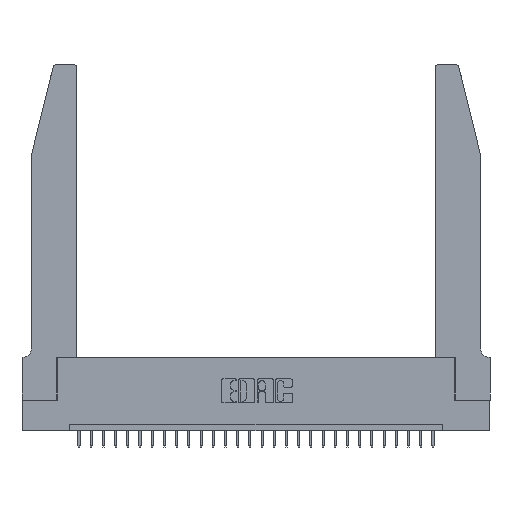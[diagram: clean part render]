
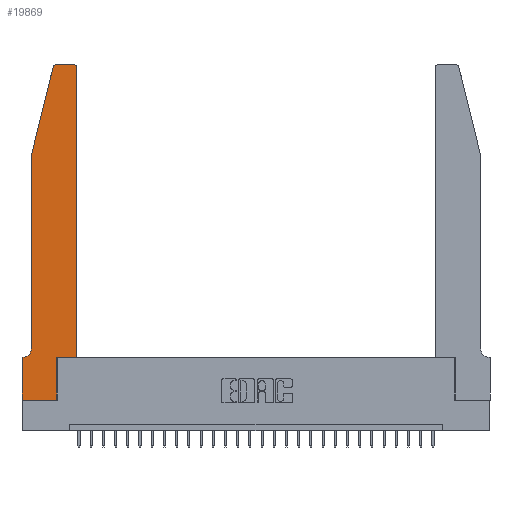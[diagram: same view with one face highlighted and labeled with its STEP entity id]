
A CAD part, top view. The second image highlights one B-rep face of the part: STEP entity #19869.
In plain terms, the highlighted planar face has unit normal (0, 0, 1).
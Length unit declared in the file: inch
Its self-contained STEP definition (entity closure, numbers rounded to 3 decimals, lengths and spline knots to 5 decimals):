
#44 = DIRECTION ( 'NONE',  ( 0., 0., 1. ) ) ;
#77 = AXIS2_PLACEMENT_3D ( 'NONE', #23384, #14602, #3394 ) ;
#98 = VECTOR ( 'NONE', #6298, 39.37008 ) ;
#285 = EDGE_CURVE ( 'NONE', #10634, #1515, #1012, .T. ) ;
#1012 = LINE ( 'NONE', #17188, #25601 ) ;
#1512 = EDGE_CURVE ( 'NONE', #27253, #10078, #5974, .T. ) ;
#1515 = VERTEX_POINT ( 'NONE', #17982 ) ;
#2240 = CARTESIAN_POINT ( 'NONE',  ( 0.284, 2.72, 0.37 ) ) ;
#2306 = ORIENTED_EDGE ( 'NONE', *, *, #8383, .T. ) ;
#2870 = CARTESIAN_POINT ( 'NONE',  ( 0.0055, 0.42, 0.37 ) ) ;
#3179 = DIRECTION ( 'NONE',  ( -0.239, -0.971, 0. ) ) ;
#3394 = DIRECTION ( 'NONE',  ( 1., 0., 0. ) ) ;
#3932 = LINE ( 'NONE', #19424, #98 ) ;
#4130 = ORIENTED_EDGE ( 'NONE', *, *, #18669, .T. ) ;
#4295 = CARTESIAN_POINT ( 'NONE',  ( 0.2865, 0.35, 0.37 ) ) ;
#4354 = ORIENTED_EDGE ( 'NONE', *, *, #24389, .T. ) ;
#4366 = EDGE_LOOP ( 'NONE', ( #11597, #15794, #4354, #13078, #4130, #20273, #5913, #2306, #17979, #25683, #22685, #17369 ) ) ;
#4673 = LINE ( 'NONE', #11327, #28421 ) ;
#5913 = ORIENTED_EDGE ( 'NONE', *, *, #285, .T. ) ;
#5974 = CIRCLE ( 'NONE', #15387, 0.03 ) ;
#6171 = VECTOR ( 'NONE', #3179, 39.37008 ) ;
#6240 = CARTESIAN_POINT ( 'NONE',  ( 0., 0., 0.37 ) ) ;
#6298 = DIRECTION ( 'NONE',  ( -1., 0., 0. ) ) ;
#7006 = DIRECTION ( 'NONE',  ( 1., 0., 0. ) ) ;
#7456 = DIRECTION ( 'NONE',  ( -1., 0., 0. ) ) ;
#7613 = CARTESIAN_POINT ( 'NONE',  ( 0.25487, 2.72718, 0.37 ) ) ;
#7630 = CARTESIAN_POINT ( 'NONE',  ( 0.284, 2.75, 0.37 ) ) ;
#7729 = CARTESIAN_POINT ( 'NONE',  ( 0.2865, 0.35, 0.37 ) ) ;
#7946 = VERTEX_POINT ( 'NONE', #17077 ) ;
#8383 = EDGE_CURVE ( 'NONE', #1515, #21923, #10683, .T. ) ;
#8468 = LINE ( 'NONE', #21669, #19269 ) ;
#8568 = DIRECTION ( 'NONE',  ( 1., 0., 0. ) ) ;
#8929 = LINE ( 'NONE', #14067, #26870 ) ;
#9000 = AXIS2_PLACEMENT_3D ( 'NONE', #19307, #28690, #8568 ) ;
#9017 = DIRECTION ( 'NONE',  ( 1., 0., 0. ) ) ;
#9411 = EDGE_CURVE ( 'NONE', #7946, #10634, #4673, .T. ) ;
#9522 = CARTESIAN_POINT ( 'NONE',  ( 0.4505, 0.35, 0.37 ) ) ;
#9962 = LINE ( 'NONE', #25504, #6171 ) ;
#10078 = VERTEX_POINT ( 'NONE', #7613 ) ;
#10200 = FACE_OUTER_BOUND ( 'NONE', #4366, .T. ) ;
#10564 = CARTESIAN_POINT ( 'NONE',  ( 0.4205, 2.75, 0.37 ) ) ;
#10634 = VERTEX_POINT ( 'NONE', #13117 ) ;
#10683 = LINE ( 'NONE', #6240, #20390 ) ;
#11327 = CARTESIAN_POINT ( 'NONE',  ( 0.0755, 0.35, 0.37 ) ) ;
#11597 = ORIENTED_EDGE ( 'NONE', *, *, #20424, .T. ) ;
#11958 = CARTESIAN_POINT ( 'NONE',  ( 0.4505, 2.72, 0.37 ) ) ;
#13078 = ORIENTED_EDGE ( 'NONE', *, *, #27452, .T. ) ;
#13117 = CARTESIAN_POINT ( 'NONE',  ( 0., 0.35, 0.37 ) ) ;
#13248 = CARTESIAN_POINT ( 'NONE',  ( 0.2865, 0., 0.37 ) ) ;
#14067 = CARTESIAN_POINT ( 'NONE',  ( 0.4505, 0.35, 0.37 ) ) ;
#14196 = AXIS2_PLACEMENT_3D ( 'NONE', #2870, #22716, #7456 ) ;
#14602 = DIRECTION ( 'NONE',  ( 0., 0., 1. ) ) ;
#14845 = CARTESIAN_POINT ( 'NONE',  ( 0.0755, 0.42, 0.37 ) ) ;
#15387 = AXIS2_PLACEMENT_3D ( 'NONE', #2240, #44, #9017 ) ;
#15687 = LINE ( 'NONE', #4295, #17085 ) ;
#15794 = ORIENTED_EDGE ( 'NONE', *, *, #1512, .T. ) ;
#16887 = CARTESIAN_POINT ( 'NONE',  ( 0.0755, 2., 0.37 ) ) ;
#17077 = CARTESIAN_POINT ( 'NONE',  ( 0.0055, 0.35, 0.37 ) ) ;
#17085 = VECTOR ( 'NONE', #26498, 39.37008 ) ;
#17188 = CARTESIAN_POINT ( 'NONE',  ( 0., 0., 0.37 ) ) ;
#17369 = ORIENTED_EDGE ( 'NONE', *, *, #20000, .T. ) ;
#17979 = ORIENTED_EDGE ( 'NONE', *, *, #28663, .T. ) ;
#17982 = CARTESIAN_POINT ( 'NONE',  ( 0., 0., 0.37 ) ) ;
#18382 = DIRECTION ( 'NONE',  ( -1., 0., 0. ) ) ;
#18389 = VERTEX_POINT ( 'NONE', #10564 ) ;
#18669 = EDGE_CURVE ( 'NONE', #24015, #7946, #26818, .T. ) ;
#18931 = VERTEX_POINT ( 'NONE', #7729 ) ;
#19269 = VECTOR ( 'NONE', #26368, 39.37008 ) ;
#19307 = CARTESIAN_POINT ( 'NONE',  ( 0.4205, 2.72, 0.37 ) ) ;
#19424 = CARTESIAN_POINT ( 'NONE',  ( 0.2605, 2.75, 0.37 ) ) ;
#19869 = ADVANCED_FACE ( 'NONE', ( #10200 ), #21076, .T. ) ;
#20000 = EDGE_CURVE ( 'NONE', #26409, #18389, #21183, .T. ) ;
#20273 = ORIENTED_EDGE ( 'NONE', *, *, #9411, .T. ) ;
#20327 = VECTOR ( 'NONE', #21547, 39.37008 ) ;
#20390 = VECTOR ( 'NONE', #21816, 39.37008 ) ;
#20424 = EDGE_CURVE ( 'NONE', #18389, #27253, #3932, .T. ) ;
#21025 = CARTESIAN_POINT ( 'NONE',  ( 0.0755, 2., 0.37 ) ) ;
#21076 = PLANE ( 'NONE',  #77 ) ;
#21183 = CIRCLE ( 'NONE', #9000, 0.03 ) ;
#21547 = DIRECTION ( 'NONE',  ( 0., -1., 0. ) ) ;
#21669 = CARTESIAN_POINT ( 'NONE',  ( 0.4505, 0.35, 0.37 ) ) ;
#21816 = DIRECTION ( 'NONE',  ( 1., 0., 0. ) ) ;
#21923 = VERTEX_POINT ( 'NONE', #13248 ) ;
#22622 = EDGE_CURVE ( 'NONE', #28340, #26409, #8468, .T. ) ;
#22685 = ORIENTED_EDGE ( 'NONE', *, *, #22622, .T. ) ;
#22716 = DIRECTION ( 'NONE',  ( 0., 0., -1. ) ) ;
#23384 = CARTESIAN_POINT ( 'NONE',  ( 0., 0.35, 0.37 ) ) ;
#24015 = VERTEX_POINT ( 'NONE', #14845 ) ;
#24389 = EDGE_CURVE ( 'NONE', #10078, #26840, #9962, .T. ) ;
#25504 = CARTESIAN_POINT ( 'NONE',  ( 0.0755, 2., 0.37 ) ) ;
#25601 = VECTOR ( 'NONE', #26397, 39.37008 ) ;
#25683 = ORIENTED_EDGE ( 'NONE', *, *, #25729, .T. ) ;
#25729 = EDGE_CURVE ( 'NONE', #18931, #28340, #8929, .T. ) ;
#26254 = LINE ( 'NONE', #16887, #20327 ) ;
#26368 = DIRECTION ( 'NONE',  ( 0., 1., 0. ) ) ;
#26397 = DIRECTION ( 'NONE',  ( 0., -1., 0. ) ) ;
#26409 = VERTEX_POINT ( 'NONE', #11958 ) ;
#26498 = DIRECTION ( 'NONE',  ( 0., 1., 0. ) ) ;
#26818 = CIRCLE ( 'NONE', #14196, 0.07 ) ;
#26840 = VERTEX_POINT ( 'NONE', #21025 ) ;
#26870 = VECTOR ( 'NONE', #7006, 39.37008 ) ;
#27253 = VERTEX_POINT ( 'NONE', #7630 ) ;
#27452 = EDGE_CURVE ( 'NONE', #26840, #24015, #26254, .T. ) ;
#28340 = VERTEX_POINT ( 'NONE', #9522 ) ;
#28421 = VECTOR ( 'NONE', #18382, 39.37008 ) ;
#28663 = EDGE_CURVE ( 'NONE', #21923, #18931, #15687, .T. ) ;
#28690 = DIRECTION ( 'NONE',  ( 0., 0., 1. ) ) ;
